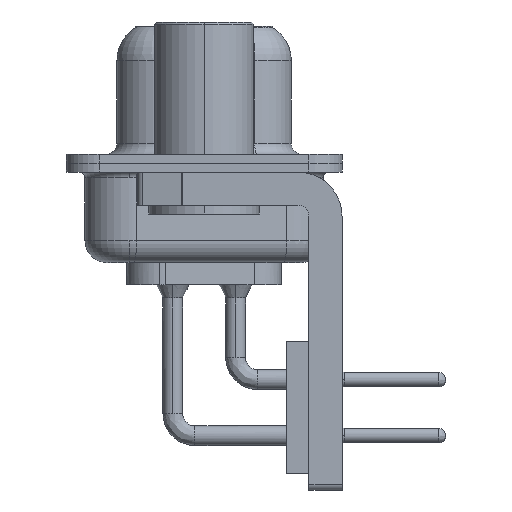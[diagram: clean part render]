
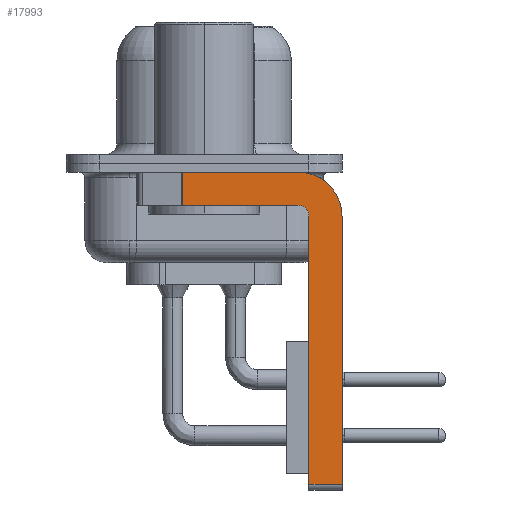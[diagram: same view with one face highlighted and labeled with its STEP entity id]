
A CAD part, left-side view. The second image highlights one B-rep face of the part: STEP entity #17993.
In plain terms, the highlighted planar face has unit normal (-1, 0, 0).
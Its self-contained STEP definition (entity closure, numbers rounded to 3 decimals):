
#228 = ORIENTED_EDGE ( 'NONE', *, *, #2595, .F. ) ;
#882 = LINE ( 'NONE', #4360, #21481 ) ;
#1214 = CARTESIAN_POINT ( 'NONE',  ( -2.9, -4.75, -14.8 ) ) ;
#1463 = DIRECTION ( 'NONE',  ( 0., -1., 0. ) ) ;
#2027 = AXIS2_PLACEMENT_3D ( 'NONE', #16749, #22650, #10965 ) ;
#2156 = VERTEX_POINT ( 'NONE', #19328 ) ;
#2200 = DIRECTION ( 'NONE',  ( 0., 0., -1. ) ) ;
#2595 = EDGE_CURVE ( 'NONE', #4996, #22777, #11302, .T. ) ;
#2671 = LINE ( 'NONE', #7487, #21285 ) ;
#3134 = ORIENTED_EDGE ( 'NONE', *, *, #16551, .T. ) ;
#3231 = ORIENTED_EDGE ( 'NONE', *, *, #15177, .F. ) ;
#3594 = CARTESIAN_POINT ( 'NONE',  ( -2.9, -4.25, -14.55 ) ) ;
#3908 = VERTEX_POINT ( 'NONE', #19372 ) ;
#4201 = DIRECTION ( 'NONE',  ( 0., 1., 0. ) ) ;
#4360 = CARTESIAN_POINT ( 'NONE',  ( -2.9, 0.978, -1.9 ) ) ;
#4499 = VERTEX_POINT ( 'NONE', #9366 ) ;
#4608 = EDGE_CURVE ( 'NONE', #2156, #4499, #17578, .T. ) ;
#4714 = VERTEX_POINT ( 'NONE', #11810 ) ;
#4996 = VERTEX_POINT ( 'NONE', #5585 ) ;
#5426 = DIRECTION ( 'NONE',  ( 0., 0., -1. ) ) ;
#5584 = EDGE_LOOP ( 'NONE', ( #25041, #7038, #228, #6558, #3231, #3134, #11349, #8221 ) ) ;
#5585 = CARTESIAN_POINT ( 'NONE',  ( -2.9, -4.25, -1.9 ) ) ;
#5911 = DIRECTION ( 'NONE',  ( -1., 0., 0. ) ) ;
#6558 = ORIENTED_EDGE ( 'NONE', *, *, #11730, .F. ) ;
#7038 = ORIENTED_EDGE ( 'NONE', *, *, #21694, .T. ) ;
#7487 = CARTESIAN_POINT ( 'NONE',  ( -2.9, -6.25, -2.4 ) ) ;
#7748 = CARTESIAN_POINT ( 'NONE',  ( -2.9, 0.978, -1.9 ) ) ;
#8221 = ORIENTED_EDGE ( 'NONE', *, *, #8234, .F. ) ;
#8234 = EDGE_CURVE ( 'NONE', #4499, #11214, #12305, .T. ) ;
#8432 = DIRECTION ( 'NONE',  ( 1., 0., 0. ) ) ;
#9366 = CARTESIAN_POINT ( 'NONE',  ( -2.9, -4.25, -0.4 ) ) ;
#10273 = AXIS2_PLACEMENT_3D ( 'NONE', #20018, #8432, #22095 ) ;
#10965 = DIRECTION ( 'NONE',  ( 0., 0., -1. ) ) ;
#11112 = VERTEX_POINT ( 'NONE', #13215 ) ;
#11214 = VERTEX_POINT ( 'NONE', #23396 ) ;
#11302 = LINE ( 'NONE', #19382, #20274 ) ;
#11349 = ORIENTED_EDGE ( 'NONE', *, *, #14530, .F. ) ;
#11730 = EDGE_CURVE ( 'NONE', #11112, #4996, #23122, .T. ) ;
#11810 = CARTESIAN_POINT ( 'NONE',  ( -2.9, -6.25, -14.55 ) ) ;
#12305 = CIRCLE ( 'NONE', #10273, 2. ) ;
#12784 = AXIS2_PLACEMENT_3D ( 'NONE', #17713, #5911, #19570 ) ;
#13215 = CARTESIAN_POINT ( 'NONE',  ( -2.9, -4.75, -2.4 ) ) ;
#14378 = VECTOR ( 'NONE', #25321, 1000. ) ;
#14530 = EDGE_CURVE ( 'NONE', #11214, #4714, #2671, .T. ) ;
#15177 = EDGE_CURVE ( 'NONE', #3908, #11112, #24891, .T. ) ;
#16551 = EDGE_CURVE ( 'NONE', #3908, #4714, #17332, .T. ) ;
#16749 = CARTESIAN_POINT ( 'NONE',  ( -2.9, -4.25, -2.4 ) ) ;
#17332 = LINE ( 'NONE', #3594, #21849 ) ;
#17578 = LINE ( 'NONE', #18029, #22819 ) ;
#17713 = CARTESIAN_POINT ( 'NONE',  ( -2.9, -4.25, -2.4 ) ) ;
#17948 = DIRECTION ( 'NONE',  ( 0., -1., 0. ) ) ;
#17993 = ADVANCED_FACE ( 'NONE', ( #24633 ), #20521, .F. ) ;
#18029 = CARTESIAN_POINT ( 'NONE',  ( -2.9, 3., -0.4 ) ) ;
#19328 = CARTESIAN_POINT ( 'NONE',  ( -2.9, 0.978, -0.4 ) ) ;
#19372 = CARTESIAN_POINT ( 'NONE',  ( -2.9, -4.75, -14.55 ) ) ;
#19382 = CARTESIAN_POINT ( 'NONE',  ( -2.9, -4.25, -1.9 ) ) ;
#19570 = DIRECTION ( 'NONE',  ( 0., 0., 1. ) ) ;
#20018 = CARTESIAN_POINT ( 'NONE',  ( -2.9, -4.25, -2.4 ) ) ;
#20274 = VECTOR ( 'NONE', #4201, 1000. ) ;
#20521 = PLANE ( 'NONE',  #2027 ) ;
#21285 = VECTOR ( 'NONE', #5426, 1000. ) ;
#21481 = VECTOR ( 'NONE', #2200, 1000. ) ;
#21694 = EDGE_CURVE ( 'NONE', #2156, #22777, #882, .T. ) ;
#21849 = VECTOR ( 'NONE', #1463, 1000. ) ;
#22095 = DIRECTION ( 'NONE',  ( 0., 0., -1. ) ) ;
#22650 = DIRECTION ( 'NONE',  ( 1., 0., 0. ) ) ;
#22777 = VERTEX_POINT ( 'NONE', #7748 ) ;
#22819 = VECTOR ( 'NONE', #17948, 1000. ) ;
#23122 = CIRCLE ( 'NONE', #12784, 0.5 ) ;
#23396 = CARTESIAN_POINT ( 'NONE',  ( -2.9, -6.25, -2.4 ) ) ;
#24633 = FACE_OUTER_BOUND ( 'NONE', #5584, .T. ) ;
#24891 = LINE ( 'NONE', #1214, #14378 ) ;
#25041 = ORIENTED_EDGE ( 'NONE', *, *, #4608, .F. ) ;
#25321 = DIRECTION ( 'NONE',  ( 0., 0., 1. ) ) ;
